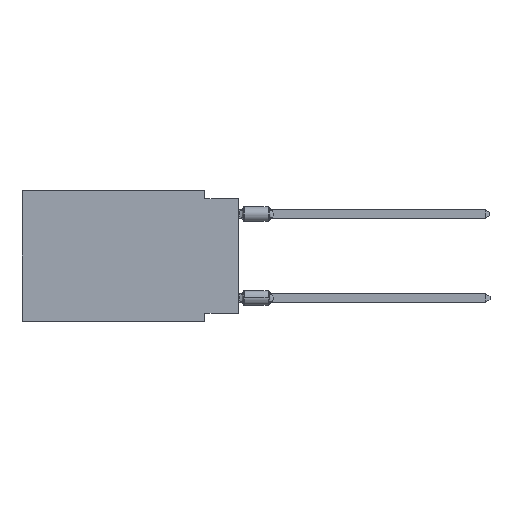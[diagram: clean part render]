
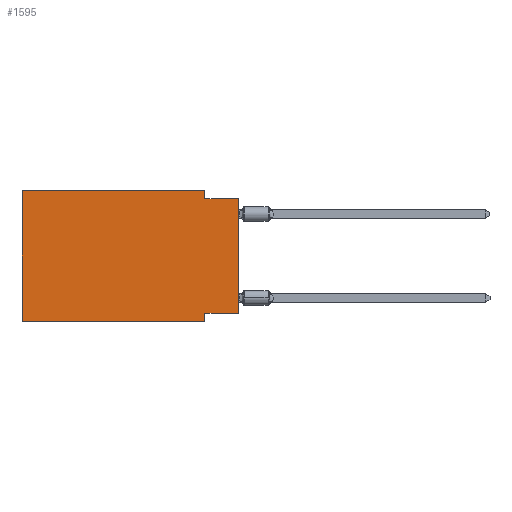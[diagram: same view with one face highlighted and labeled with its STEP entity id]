
A CAD part, left-side view. The second image highlights one B-rep face of the part: STEP entity #1595.
In plain terms, the highlighted planar face has unit normal (-1, 0, 0).
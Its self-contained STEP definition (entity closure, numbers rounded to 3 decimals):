
#77 = ORIENTED_EDGE ( 'NONE', *, *, #27753, .T. ) ;
#200 = DIRECTION ( 'NONE',  ( 0., -1., 0. ) ) ;
#1276 = CARTESIAN_POINT ( 'NONE',  ( 0., 16.383, 0. ) ) ;
#1354 = CARTESIAN_POINT ( 'NONE',  ( 0., 0., -9.271 ) ) ;
#1595 = ADVANCED_FACE ( 'NONE', ( #27819 ), #14340, .F. ) ;
#1675 = CARTESIAN_POINT ( 'NONE',  ( 0., 16.383, -9.906 ) ) ;
#1947 = EDGE_CURVE ( 'NONE', #10852, #26950, #27894, .T. ) ;
#2073 = CARTESIAN_POINT ( 'NONE',  ( 0., 16.383, 0. ) ) ;
#2282 = VERTEX_POINT ( 'NONE', #5667 ) ;
#2351 = CARTESIAN_POINT ( 'NONE',  ( 0., 16.383, 0. ) ) ;
#2889 = CARTESIAN_POINT ( 'NONE',  ( 0., 0., -9.271 ) ) ;
#3586 = EDGE_CURVE ( 'NONE', #7125, #6739, #20010, .T. ) ;
#5667 = CARTESIAN_POINT ( 'NONE',  ( 0., 2.54, -9.906 ) ) ;
#5865 = AXIS2_PLACEMENT_3D ( 'NONE', #1276, #18656, #16917 ) ;
#6650 = VECTOR ( 'NONE', #200, 1000. ) ;
#6739 = VERTEX_POINT ( 'NONE', #27251 ) ;
#7125 = VERTEX_POINT ( 'NONE', #11591 ) ;
#7652 = LINE ( 'NONE', #22898, #20210 ) ;
#7677 = CARTESIAN_POINT ( 'NONE',  ( 0., 2.54, -0.635 ) ) ;
#8897 = ORIENTED_EDGE ( 'NONE', *, *, #3586, .F. ) ;
#9084 = CARTESIAN_POINT ( 'NONE',  ( 0., 0., 0. ) ) ;
#9155 = EDGE_CURVE ( 'NONE', #27067, #7125, #28036, .T. ) ;
#9713 = DIRECTION ( 'NONE',  ( 0., 0., -1. ) ) ;
#9847 = CARTESIAN_POINT ( 'NONE',  ( 0., 2.54, 0. ) ) ;
#9888 = VERTEX_POINT ( 'NONE', #27263 ) ;
#9984 = LINE ( 'NONE', #9847, #17910 ) ;
#10852 = VERTEX_POINT ( 'NONE', #2889 ) ;
#11493 = EDGE_CURVE ( 'NONE', #27067, #2282, #26211, .T. ) ;
#11591 = CARTESIAN_POINT ( 'NONE',  ( 0., 16.383, 0. ) ) ;
#12133 = ORIENTED_EDGE ( 'NONE', *, *, #11493, .T. ) ;
#14340 = PLANE ( 'NONE',  #5865 ) ;
#14446 = ORIENTED_EDGE ( 'NONE', *, *, #22108, .F. ) ;
#14790 = CARTESIAN_POINT ( 'NONE',  ( 0., 0., -0.635 ) ) ;
#15608 = VECTOR ( 'NONE', #23796, 1000. ) ;
#15656 = EDGE_CURVE ( 'NONE', #26950, #2282, #7652, .T. ) ;
#15697 = ORIENTED_EDGE ( 'NONE', *, *, #27002, .F. ) ;
#16242 = ORIENTED_EDGE ( 'NONE', *, *, #9155, .F. ) ;
#16917 = DIRECTION ( 'NONE',  ( 0., 0., -1. ) ) ;
#17910 = VECTOR ( 'NONE', #9713, 1000. ) ;
#17986 = DIRECTION ( 'NONE',  ( 0., 0., 1. ) ) ;
#18264 = LINE ( 'NONE', #9084, #27429 ) ;
#18656 = DIRECTION ( 'NONE',  ( 1., 0., 0. ) ) ;
#20010 = LINE ( 'NONE', #2073, #6650 ) ;
#20210 = VECTOR ( 'NONE', #22482, 1000. ) ;
#21311 = DIRECTION ( 'NONE',  ( 0., 1., 0. ) ) ;
#21687 = CARTESIAN_POINT ( 'NONE',  ( 0., 2.54, -9.271 ) ) ;
#22108 = EDGE_CURVE ( 'NONE', #25889, #9888, #27847, .T. ) ;
#22482 = DIRECTION ( 'NONE',  ( 0., 0., -1. ) ) ;
#22898 = CARTESIAN_POINT ( 'NONE',  ( 0., 2.54, -9.906 ) ) ;
#23056 = CARTESIAN_POINT ( 'NONE',  ( 0., 16.383, -9.906 ) ) ;
#23422 = DIRECTION ( 'NONE',  ( 0., -1., 0. ) ) ;
#23747 = DIRECTION ( 'NONE',  ( 0., 0., 1. ) ) ;
#23768 = VECTOR ( 'NONE', #21311, 1000. ) ;
#23796 = DIRECTION ( 'NONE',  ( 0., -1., 0. ) ) ;
#25875 = VECTOR ( 'NONE', #23422, 1000. ) ;
#25889 = VERTEX_POINT ( 'NONE', #7677 ) ;
#26211 = LINE ( 'NONE', #1675, #15608 ) ;
#26296 = ORIENTED_EDGE ( 'NONE', *, *, #15656, .F. ) ;
#26950 = VERTEX_POINT ( 'NONE', #21687 ) ;
#27002 = EDGE_CURVE ( 'NONE', #6739, #25889, #9984, .T. ) ;
#27067 = VERTEX_POINT ( 'NONE', #23056 ) ;
#27251 = CARTESIAN_POINT ( 'NONE',  ( 0., 2.54, 0. ) ) ;
#27263 = CARTESIAN_POINT ( 'NONE',  ( 0., 0., -0.635 ) ) ;
#27297 = EDGE_LOOP ( 'NONE', ( #77, #14446, #15697, #8897, #16242, #12133, #26296, #28106 ) ) ;
#27429 = VECTOR ( 'NONE', #17986, 1000. ) ;
#27753 = EDGE_CURVE ( 'NONE', #10852, #9888, #18264, .T. ) ;
#27819 = FACE_OUTER_BOUND ( 'NONE', #27297, .T. ) ;
#27847 = LINE ( 'NONE', #14790, #25875 ) ;
#27894 = LINE ( 'NONE', #1354, #23768 ) ;
#28036 = LINE ( 'NONE', #2351, #28334 ) ;
#28106 = ORIENTED_EDGE ( 'NONE', *, *, #1947, .F. ) ;
#28334 = VECTOR ( 'NONE', #23747, 1000. ) ;
